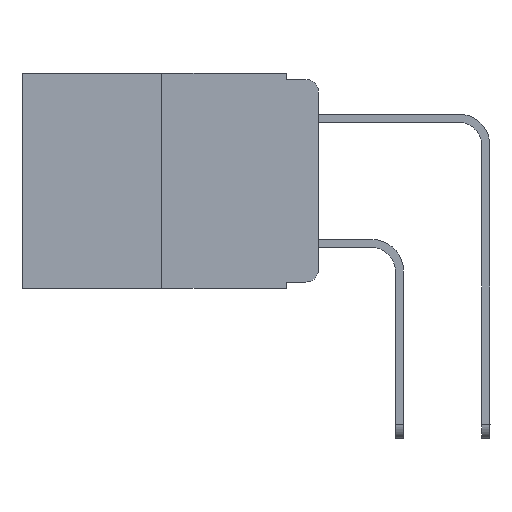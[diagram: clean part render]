
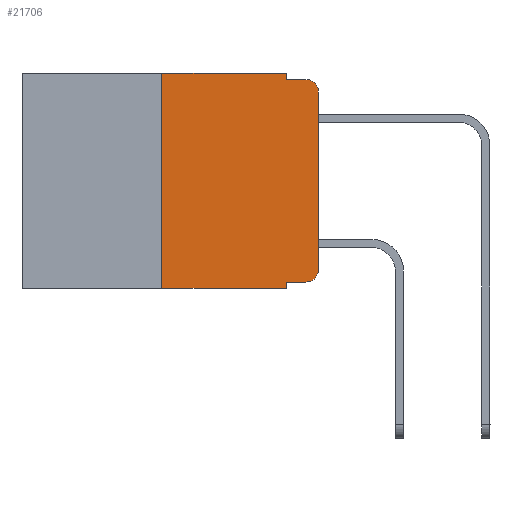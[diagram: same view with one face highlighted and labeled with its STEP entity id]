
A CAD part, left-side view. The second image highlights one B-rep face of the part: STEP entity #21706.
In plain terms, the highlighted planar face has unit normal (-1, 0, 0).
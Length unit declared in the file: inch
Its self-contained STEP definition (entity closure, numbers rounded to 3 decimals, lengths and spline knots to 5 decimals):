
#748 = CIRCLE ( 'NONE', #21151, 0.02 ) ;
#772 = EDGE_CURVE ( 'NONE', #4326, #10841, #12421, .T. ) ;
#907 = CARTESIAN_POINT ( 'NONE',  ( 0., 0.051, 0. ) ) ;
#993 = CARTESIAN_POINT ( 'NONE',  ( 0., 0.051, 0. ) ) ;
#1214 = EDGE_CURVE ( 'NONE', #14583, #11067, #24385, .T. ) ;
#1304 = AXIS2_PLACEMENT_3D ( 'NONE', #1378, #3575, #25489 ) ;
#1378 = CARTESIAN_POINT ( 'NONE',  ( 0., 0.02, -0.313 ) ) ;
#2091 = VERTEX_POINT ( 'NONE', #20270 ) ;
#2108 = EDGE_CURVE ( 'NONE', #14583, #2091, #20539, .T. ) ;
#2698 = LINE ( 'NONE', #22778, #21955 ) ;
#3208 = ORIENTED_EDGE ( 'NONE', *, *, #12362, .T. ) ;
#3332 = VECTOR ( 'NONE', #5850, 39.37008 ) ;
#3375 = CIRCLE ( 'NONE', #1304, 0.02 ) ;
#3575 = DIRECTION ( 'NONE',  ( -1., 0., 0. ) ) ;
#3646 = LINE ( 'NONE', #9647, #3332 ) ;
#3680 = CARTESIAN_POINT ( 'NONE',  ( 0., 0.02, -0.01 ) ) ;
#4184 = CARTESIAN_POINT ( 'NONE',  ( 0., 0.051, -0.333 ) ) ;
#4326 = VERTEX_POINT ( 'NONE', #4184 ) ;
#4502 = VECTOR ( 'NONE', #20912, 39.37008 ) ;
#5139 = EDGE_LOOP ( 'NONE', ( #12624, #9915, #14407, #12416, #22457, #20892, #23489, #7260, #15659, #3208 ) ) ;
#5480 = CARTESIAN_POINT ( 'NONE',  ( 0., 0.473, 0. ) ) ;
#5850 = DIRECTION ( 'NONE',  ( 0., 0., 1. ) ) ;
#6810 = LINE ( 'NONE', #9154, #4502 ) ;
#7260 = ORIENTED_EDGE ( 'NONE', *, *, #22910, .F. ) ;
#7404 = VECTOR ( 'NONE', #19133, 39.37008 ) ;
#7553 = CARTESIAN_POINT ( 'NONE',  ( 0., 0.051, 0. ) ) ;
#7862 = VERTEX_POINT ( 'NONE', #14051 ) ;
#8966 = EDGE_CURVE ( 'NONE', #11067, #21253, #6810, .T. ) ;
#9148 = EDGE_CURVE ( 'NONE', #7862, #12826, #748, .T. ) ;
#9154 = CARTESIAN_POINT ( 'NONE',  ( 0., 0.473, 0. ) ) ;
#9247 = DIRECTION ( 'NONE',  ( 0., 0., -1. ) ) ;
#9647 = CARTESIAN_POINT ( 'NONE',  ( 0., 0., 0. ) ) ;
#9750 = VECTOR ( 'NONE', #9247, 39.37008 ) ;
#9915 = ORIENTED_EDGE ( 'NONE', *, *, #9148, .T. ) ;
#10101 = DIRECTION ( 'NONE',  ( 0., -1., 0. ) ) ;
#10203 = DIRECTION ( 'NONE',  ( 0., 0., 1. ) ) ;
#10364 = CARTESIAN_POINT ( 'NONE',  ( 0., 0.473, -0.343 ) ) ;
#10841 = VERTEX_POINT ( 'NONE', #12454 ) ;
#11067 = VERTEX_POINT ( 'NONE', #21686 ) ;
#11472 = DIRECTION ( 'NONE',  ( 1., 0., 0. ) ) ;
#11553 = EDGE_CURVE ( 'NONE', #12171, #7862, #3646, .T. ) ;
#12171 = VERTEX_POINT ( 'NONE', #13212 ) ;
#12348 = AXIS2_PLACEMENT_3D ( 'NONE', #5480, #11472, #19423 ) ;
#12362 = EDGE_CURVE ( 'NONE', #10841, #12171, #3375, .T. ) ;
#12416 = ORIENTED_EDGE ( 'NONE', *, *, #16852, .F. ) ;
#12421 = LINE ( 'NONE', #22100, #13888 ) ;
#12431 = DIRECTION ( 'NONE',  ( 0., -1., 0. ) ) ;
#12454 = CARTESIAN_POINT ( 'NONE',  ( 0., 0.02, -0.333 ) ) ;
#12624 = ORIENTED_EDGE ( 'NONE', *, *, #11553, .T. ) ;
#12826 = VERTEX_POINT ( 'NONE', #3680 ) ;
#13212 = CARTESIAN_POINT ( 'NONE',  ( 0., 0., -0.313 ) ) ;
#13673 = PLANE ( 'NONE',  #12348 ) ;
#13888 = VECTOR ( 'NONE', #10101, 39.37008 ) ;
#14051 = CARTESIAN_POINT ( 'NONE',  ( 0., 0., -0.03 ) ) ;
#14407 = ORIENTED_EDGE ( 'NONE', *, *, #18532, .F. ) ;
#14583 = VERTEX_POINT ( 'NONE', #25567 ) ;
#15396 = FACE_OUTER_BOUND ( 'NONE', #5139, .T. ) ;
#15659 = ORIENTED_EDGE ( 'NONE', *, *, #772, .T. ) ;
#16852 = EDGE_CURVE ( 'NONE', #21253, #23661, #23327, .T. ) ;
#18532 = EDGE_CURVE ( 'NONE', #23661, #12826, #2698, .T. ) ;
#18669 = CARTESIAN_POINT ( 'NONE',  ( 0., 0.051, -0.01 ) ) ;
#18688 = VECTOR ( 'NONE', #10203, 39.37008 ) ;
#19133 = DIRECTION ( 'NONE',  ( 0., 0., -1. ) ) ;
#19423 = DIRECTION ( 'NONE',  ( 0., 0., -1. ) ) ;
#19847 = CARTESIAN_POINT ( 'NONE',  ( 0., 0.02, -0.03 ) ) ;
#20270 = CARTESIAN_POINT ( 'NONE',  ( 0., 0.051, -0.343 ) ) ;
#20539 = LINE ( 'NONE', #10364, #24761 ) ;
#20892 = ORIENTED_EDGE ( 'NONE', *, *, #1214, .F. ) ;
#20912 = DIRECTION ( 'NONE',  ( 0., -1., 0. ) ) ;
#21151 = AXIS2_PLACEMENT_3D ( 'NONE', #19847, #21440, #25330 ) ;
#21253 = VERTEX_POINT ( 'NONE', #993 ) ;
#21440 = DIRECTION ( 'NONE',  ( -1., 0., 0. ) ) ;
#21686 = CARTESIAN_POINT ( 'NONE',  ( 0., 0.25, 0. ) ) ;
#21706 = ADVANCED_FACE ( 'NONE', ( #15396 ), #13673, .F. ) ;
#21951 = CARTESIAN_POINT ( 'NONE',  ( 0., 0.25, 0. ) ) ;
#21955 = VECTOR ( 'NONE', #22907, 39.37008 ) ;
#22100 = CARTESIAN_POINT ( 'NONE',  ( 0., 0.051, -0.333 ) ) ;
#22457 = ORIENTED_EDGE ( 'NONE', *, *, #8966, .F. ) ;
#22778 = CARTESIAN_POINT ( 'NONE',  ( 0., 0.051, -0.01 ) ) ;
#22795 = LINE ( 'NONE', #907, #7404 ) ;
#22907 = DIRECTION ( 'NONE',  ( 0., -1., 0. ) ) ;
#22910 = EDGE_CURVE ( 'NONE', #4326, #2091, #22795, .T. ) ;
#23327 = LINE ( 'NONE', #7553, #9750 ) ;
#23489 = ORIENTED_EDGE ( 'NONE', *, *, #2108, .T. ) ;
#23661 = VERTEX_POINT ( 'NONE', #18669 ) ;
#24385 = LINE ( 'NONE', #21951, #18688 ) ;
#24761 = VECTOR ( 'NONE', #12431, 39.37008 ) ;
#25330 = DIRECTION ( 'NONE',  ( 0., 0., -1. ) ) ;
#25489 = DIRECTION ( 'NONE',  ( 0., 0., -1. ) ) ;
#25567 = CARTESIAN_POINT ( 'NONE',  ( 0., 0.25, -0.343 ) ) ;
